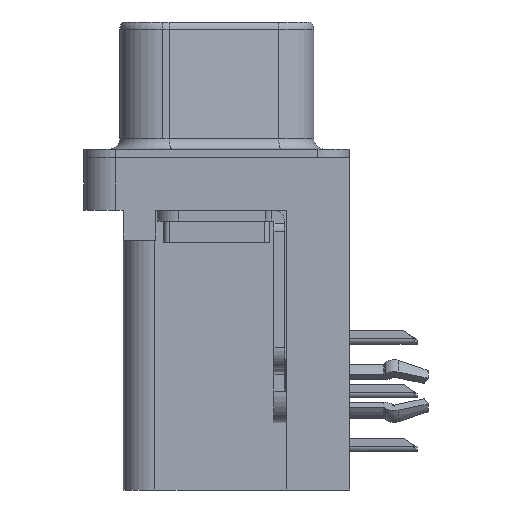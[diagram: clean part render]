
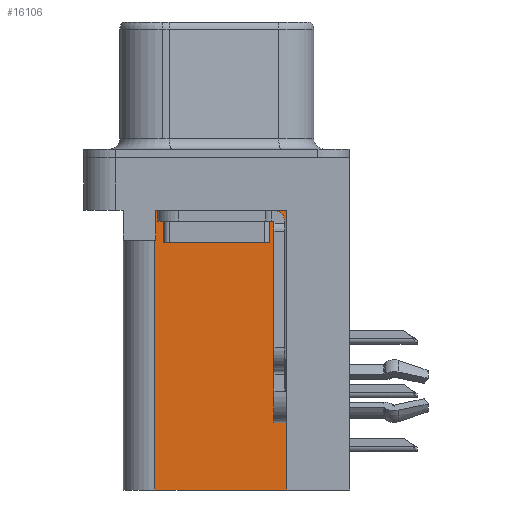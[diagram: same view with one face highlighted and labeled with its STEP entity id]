
A CAD part, left-side view. The second image highlights one B-rep face of the part: STEP entity #16106.
In plain terms, the highlighted planar face has unit normal (-1, 0, 0).
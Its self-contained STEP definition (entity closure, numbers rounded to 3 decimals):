
#775 = ORIENTED_EDGE ( 'NONE', *, *, #9769, .T. ) ;
#854 = CARTESIAN_POINT ( 'NONE',  ( 3.765, 2.895, -3.9 ) ) ;
#1946 = CARTESIAN_POINT ( 'NONE',  ( 3.765, 0., -3.9 ) ) ;
#2102 = VECTOR ( 'NONE', #9899, 1000. ) ;
#2169 = LINE ( 'NONE', #7821, #2102 ) ;
#2180 = VECTOR ( 'NONE', #21454, 1000. ) ;
#2376 = LINE ( 'NONE', #23287, #2180 ) ;
#4421 = CARTESIAN_POINT ( 'NONE',  ( 3.765, 2.925, -3.9 ) ) ;
#4558 = CARTESIAN_POINT ( 'NONE',  ( 3.765, -3.295, -15.7 ) ) ;
#4609 = ORIENTED_EDGE ( 'NONE', *, *, #18112, .T. ) ;
#4926 = VERTEX_POINT ( 'NONE', #4558 ) ;
#4943 = VERTEX_POINT ( 'NONE', #20446 ) ;
#5421 = DIRECTION ( 'NONE',  ( 0., 1., 0. ) ) ;
#5637 = ORIENTED_EDGE ( 'NONE', *, *, #8481, .T. ) ;
#6153 = VERTEX_POINT ( 'NONE', #19452 ) ;
#6154 = ORIENTED_EDGE ( 'NONE', *, *, #18115, .F. ) ;
#6446 = VERTEX_POINT ( 'NONE', #4421 ) ;
#6502 = VECTOR ( 'NONE', #10142, 1000. ) ;
#6510 = LINE ( 'NONE', #1946, #6502 ) ;
#7821 = CARTESIAN_POINT ( 'NONE',  ( 3.765, -3.295, -15.7 ) ) ;
#8481 = EDGE_CURVE ( 'NONE', #6153, #24990, #11159, .T. ) ;
#9769 = EDGE_CURVE ( 'NONE', #24990, #6446, #6510, .T. ) ;
#9899 = DIRECTION ( 'NONE',  ( 0., 1., 0. ) ) ;
#9911 = DIRECTION ( 'NONE',  ( 1., 0., 0. ) ) ;
#9976 = FACE_OUTER_BOUND ( 'NONE', #21056, .T. ) ;
#10142 = DIRECTION ( 'NONE',  ( 0., 1., 0. ) ) ;
#11159 = LINE ( 'NONE', #854, #11211 ) ;
#11211 = VECTOR ( 'NONE', #15031, 1000. ) ;
#11365 = VERTEX_POINT ( 'NONE', #21198 ) ;
#12201 = VECTOR ( 'NONE', #24663, 1000. ) ;
#12374 = LINE ( 'NONE', #18993, #12201 ) ;
#13994 = ORIENTED_EDGE ( 'NONE', *, *, #25213, .T. ) ;
#14850 = CARTESIAN_POINT ( 'NONE',  ( 3.765, 2.895, -3.9 ) ) ;
#15031 = DIRECTION ( 'NONE',  ( 0., 0., -1. ) ) ;
#15735 = LINE ( 'NONE', #17498, #16128 ) ;
#16106 = ADVANCED_FACE ( 'NONE', ( #9976 ), #19683, .F. ) ;
#16128 = VECTOR ( 'NONE', #5421, 1000. ) ;
#17498 = CARTESIAN_POINT ( 'NONE',  ( 3.765, -3.295, -2.5 ) ) ;
#18112 = EDGE_CURVE ( 'NONE', #4926, #4943, #2376, .T. ) ;
#18115 = EDGE_CURVE ( 'NONE', #4926, #11365, #2169, .T. ) ;
#18993 = CARTESIAN_POINT ( 'NONE',  ( 3.765, 2.925, -15.7 ) ) ;
#19452 = CARTESIAN_POINT ( 'NONE',  ( 3.765, 2.895, -2.5 ) ) ;
#19683 = PLANE ( 'NONE',  #24770 ) ;
#20446 = CARTESIAN_POINT ( 'NONE',  ( 3.765, -3.295, -2.5 ) ) ;
#21056 = EDGE_LOOP ( 'NONE', ( #13994, #5637, #775, #21085, #6154, #4609 ) ) ;
#21085 = ORIENTED_EDGE ( 'NONE', *, *, #25543, .F. ) ;
#21198 = CARTESIAN_POINT ( 'NONE',  ( 3.765, 2.925, -15.7 ) ) ;
#21454 = DIRECTION ( 'NONE',  ( 0., 0., 1. ) ) ;
#21545 = CARTESIAN_POINT ( 'NONE',  ( 3.765, -3.295, -15.7 ) ) ;
#23287 = CARTESIAN_POINT ( 'NONE',  ( 3.765, -3.295, -15.7 ) ) ;
#23380 = DIRECTION ( 'NONE',  ( 0., 0., -1. ) ) ;
#24663 = DIRECTION ( 'NONE',  ( 0., 0., 1. ) ) ;
#24770 = AXIS2_PLACEMENT_3D ( 'NONE', #21545, #9911, #23380 ) ;
#24990 = VERTEX_POINT ( 'NONE', #14850 ) ;
#25213 = EDGE_CURVE ( 'NONE', #4943, #6153, #15735, .T. ) ;
#25543 = EDGE_CURVE ( 'NONE', #11365, #6446, #12374, .T. ) ;
